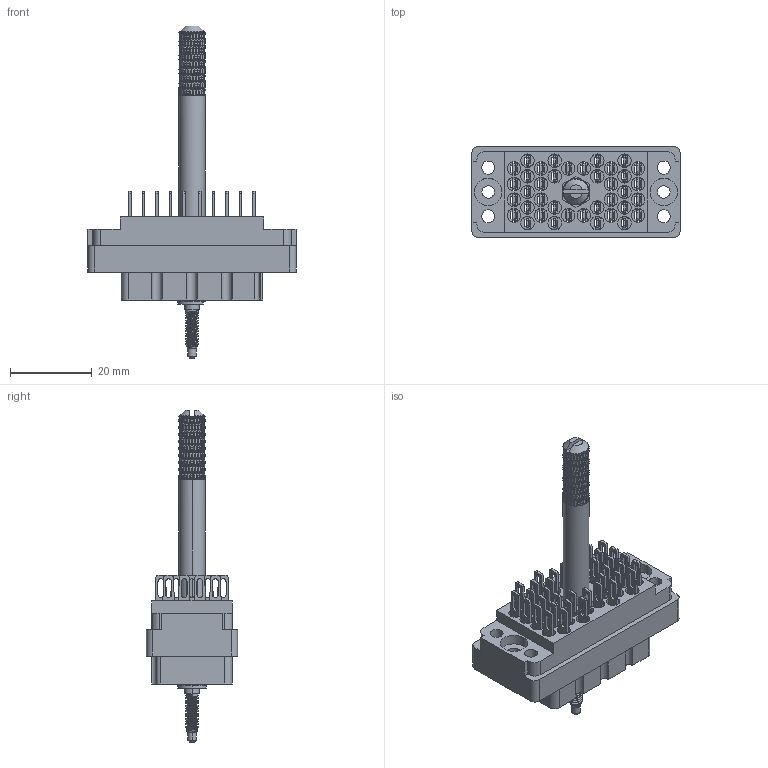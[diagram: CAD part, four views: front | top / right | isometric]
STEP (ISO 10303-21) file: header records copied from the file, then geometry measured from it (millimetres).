
FILE_DESCRIPTION (( 'STEP AP203' ), '1' );
FILE_NAME ('516-038-500-405.STEP', '2020-03-05T12:04:59', ( '' ), ( '' ), 'SwSTEP 2.0', 'SolidWorks 2016', '' );
FILE_SCHEMA (( 'CONFIG_CONTROL_DESIGN' ));
Length unit declared in the file: inch
Products named in the file (8): 516-253-138-107; 516-250-038-111; 516-292-001_500 Contact; Actuating Screw Assy 038-056; 516-251-035-100; 516-038-500-405; 516 Part Receptacle_038; 516-253-035-100
Assembly tree (45 placements, depth 3):
  516-038-500-405
    516 Part Receptacle_038
    516-292-001_500 Contact  x38
    Actuating Screw Assy 038-056
      516-251-035-100
      516-253-035-100  x2
      516-253-138-107
      516-250-038-111
Bounding box: 50.8 x 22.25 x 81.03 mm (x, y, z)
Volume: 14027.7 mm3; surface area: 23382.9 mm2
Topology: 44 solids, 44 shells, 5205 faces, 14056 edges, 8958 vertices
Faces by surface type: plane 2347, cylinder 1604, bspline 1234, cone 20
Entity records: 101691 total; most frequent: CARTESIAN_POINT 54336, ORIENTED_EDGE 11808, DIRECTION 6998, EDGE_CURVE 5904, VERTEX_POINT 3548, EDGE_LOOP 2504, ADVANCED_FACE 2387, FACE_OUTER_BOUND 2387
